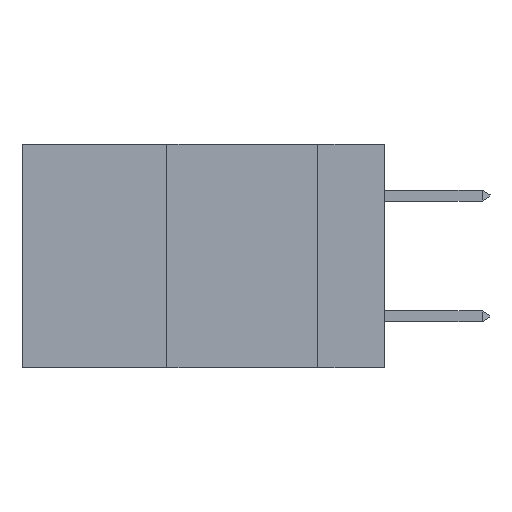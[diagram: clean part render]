
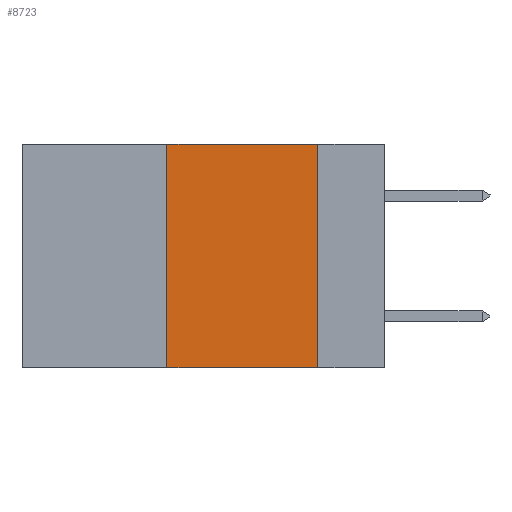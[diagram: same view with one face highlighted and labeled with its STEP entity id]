
A CAD part, left-side view. The second image highlights one B-rep face of the part: STEP entity #8723.
In plain terms, the highlighted planar face has unit normal (-1, 0, 0).
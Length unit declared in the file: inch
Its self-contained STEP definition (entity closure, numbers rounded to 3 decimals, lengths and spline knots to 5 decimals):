
#437 = VERTEX_POINT ( 'NONE', #13631 ) ;
#554 = LINE ( 'NONE', #5707, #3554 ) ;
#663 = AXIS2_PLACEMENT_3D ( 'NONE', #9869, #2962, #10949 ) ;
#2904 = PLANE ( 'NONE',  #663 ) ;
#2962 = DIRECTION ( 'NONE',  ( 1., 0., 0. ) ) ;
#3446 = EDGE_CURVE ( 'NONE', #7508, #5919, #6026, .T. ) ;
#3554 = VECTOR ( 'NONE', #11277, 39.37008 ) ;
#3663 = VECTOR ( 'NONE', #8593, 39.37008 ) ;
#3751 = FACE_OUTER_BOUND ( 'NONE', #10476, .T. ) ;
#3965 = CARTESIAN_POINT ( 'NONE',  ( 0., 0.36, -0.37 ) ) ;
#4287 = CARTESIAN_POINT ( 'NONE',  ( 0., 0.11, 0. ) ) ;
#5222 = ORIENTED_EDGE ( 'NONE', *, *, #11070, .F. ) ;
#5707 = CARTESIAN_POINT ( 'NONE',  ( 0., 0.11, 0. ) ) ;
#5919 = VERTEX_POINT ( 'NONE', #4287 ) ;
#5927 = LINE ( 'NONE', #14436, #11155 ) ;
#6026 = LINE ( 'NONE', #7160, #8696 ) ;
#6342 = ORIENTED_EDGE ( 'NONE', *, *, #14560, .T. ) ;
#7160 = CARTESIAN_POINT ( 'NONE',  ( 0., 0.6, 0. ) ) ;
#7508 = VERTEX_POINT ( 'NONE', #8356 ) ;
#8356 = CARTESIAN_POINT ( 'NONE',  ( 0., 0.36, 0. ) ) ;
#8593 = DIRECTION ( 'NONE',  ( 0., -1., 0. ) ) ;
#8696 = VECTOR ( 'NONE', #14733, 39.37008 ) ;
#8723 = ADVANCED_FACE ( 'NONE', ( #3751 ), #2904, .F. ) ;
#8919 = DIRECTION ( 'NONE',  ( 0., 0., 1. ) ) ;
#9784 = VERTEX_POINT ( 'NONE', #3965 ) ;
#9869 = CARTESIAN_POINT ( 'NONE',  ( 0., 0.6, 0. ) ) ;
#10476 = EDGE_LOOP ( 'NONE', ( #5222, #14902, #12808, #6342 ) ) ;
#10949 = DIRECTION ( 'NONE',  ( 0., 0., -1. ) ) ;
#11070 = EDGE_CURVE ( 'NONE', #5919, #437, #554, .T. ) ;
#11155 = VECTOR ( 'NONE', #8919, 39.37008 ) ;
#11277 = DIRECTION ( 'NONE',  ( 0., 0., -1. ) ) ;
#11854 = CARTESIAN_POINT ( 'NONE',  ( 0., 0.6, -0.37 ) ) ;
#12295 = EDGE_CURVE ( 'NONE', #9784, #7508, #5927, .T. ) ;
#12656 = LINE ( 'NONE', #11854, #3663 ) ;
#12808 = ORIENTED_EDGE ( 'NONE', *, *, #12295, .F. ) ;
#13631 = CARTESIAN_POINT ( 'NONE',  ( 0., 0.11, -0.37 ) ) ;
#14436 = CARTESIAN_POINT ( 'NONE',  ( 0., 0.36, 0. ) ) ;
#14560 = EDGE_CURVE ( 'NONE', #9784, #437, #12656, .T. ) ;
#14733 = DIRECTION ( 'NONE',  ( 0., -1., 0. ) ) ;
#14902 = ORIENTED_EDGE ( 'NONE', *, *, #3446, .F. ) ;
